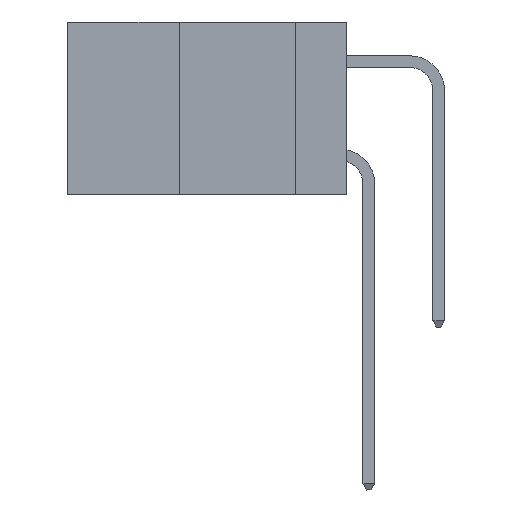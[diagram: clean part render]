
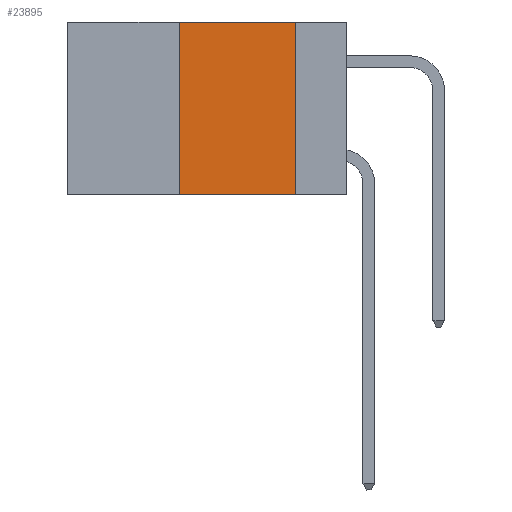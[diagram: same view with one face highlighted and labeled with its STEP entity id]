
A CAD part, left-side view. The second image highlights one B-rep face of the part: STEP entity #23895.
In plain terms, the highlighted planar face has unit normal (-1, 0, 0).
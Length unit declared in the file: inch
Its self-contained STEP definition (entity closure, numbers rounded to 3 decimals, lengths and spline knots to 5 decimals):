
#550 = DIRECTION ( 'NONE',  ( 0., 0., -1. ) ) ;
#2425 = LINE ( 'NONE', #19349, #13031 ) ;
#2951 = VECTOR ( 'NONE', #16692, 39.37008 ) ;
#3255 = CARTESIAN_POINT ( 'NONE',  ( 0., 0.36, -0.37 ) ) ;
#5424 = LINE ( 'NONE', #19851, #2951 ) ;
#5641 = EDGE_CURVE ( 'NONE', #14887, #20439, #2425, .T. ) ;
#6098 = CARTESIAN_POINT ( 'NONE',  ( 0., 0.6, 0. ) ) ;
#6404 = ORIENTED_EDGE ( 'NONE', *, *, #15152, .F. ) ;
#7306 = DIRECTION ( 'NONE',  ( 0., -1., 0. ) ) ;
#8437 = PLANE ( 'NONE',  #9587 ) ;
#9587 = AXIS2_PLACEMENT_3D ( 'NONE', #22244, #12430, #550 ) ;
#12430 = DIRECTION ( 'NONE',  ( 1., 0., 0. ) ) ;
#13031 = VECTOR ( 'NONE', #15265, 39.37008 ) ;
#14010 = LINE ( 'NONE', #6098, #16779 ) ;
#14826 = VECTOR ( 'NONE', #17125, 39.37008 ) ;
#14887 = VERTEX_POINT ( 'NONE', #3255 ) ;
#15121 = VERTEX_POINT ( 'NONE', #19915 ) ;
#15152 = EDGE_CURVE ( 'NONE', #20439, #15121, #14010, .T. ) ;
#15265 = DIRECTION ( 'NONE',  ( 0., 0., 1. ) ) ;
#16056 = ORIENTED_EDGE ( 'NONE', *, *, #22285, .T. ) ;
#16204 = EDGE_LOOP ( 'NONE', ( #21382, #6404, #19040, #16056 ) ) ;
#16692 = DIRECTION ( 'NONE',  ( 0., 0., -1. ) ) ;
#16779 = VECTOR ( 'NONE', #7306, 39.37008 ) ;
#17125 = DIRECTION ( 'NONE',  ( 0., -1., 0. ) ) ;
#17573 = EDGE_CURVE ( 'NONE', #15121, #21837, #5424, .T. ) ;
#18464 = LINE ( 'NONE', #19235, #14826 ) ;
#19040 = ORIENTED_EDGE ( 'NONE', *, *, #5641, .F. ) ;
#19235 = CARTESIAN_POINT ( 'NONE',  ( 0., 0.6, -0.37 ) ) ;
#19349 = CARTESIAN_POINT ( 'NONE',  ( 0., 0.36, 0. ) ) ;
#19851 = CARTESIAN_POINT ( 'NONE',  ( 0., 0.11, 0. ) ) ;
#19915 = CARTESIAN_POINT ( 'NONE',  ( 0., 0.11, 0. ) ) ;
#20439 = VERTEX_POINT ( 'NONE', #20469 ) ;
#20469 = CARTESIAN_POINT ( 'NONE',  ( 0., 0.36, 0. ) ) ;
#21382 = ORIENTED_EDGE ( 'NONE', *, *, #17573, .F. ) ;
#21570 = CARTESIAN_POINT ( 'NONE',  ( 0., 0.11, -0.37 ) ) ;
#21837 = VERTEX_POINT ( 'NONE', #21570 ) ;
#22244 = CARTESIAN_POINT ( 'NONE',  ( 0., 0.6, 0. ) ) ;
#22285 = EDGE_CURVE ( 'NONE', #14887, #21837, #18464, .T. ) ;
#23895 = ADVANCED_FACE ( 'NONE', ( #24005 ), #8437, .F. ) ;
#24005 = FACE_OUTER_BOUND ( 'NONE', #16204, .T. ) ;
